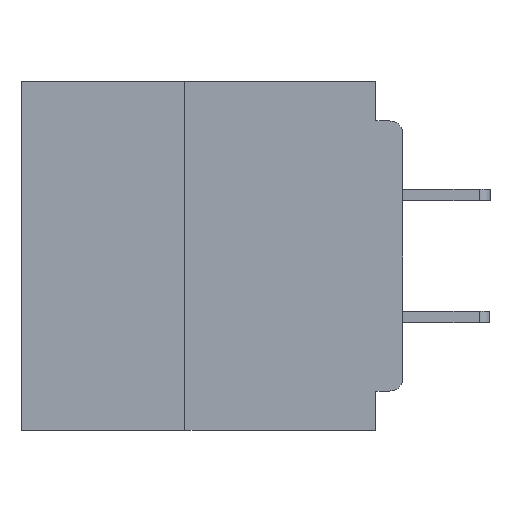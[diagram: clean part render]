
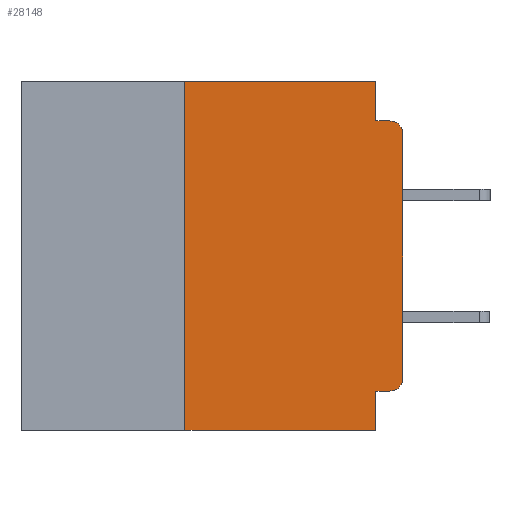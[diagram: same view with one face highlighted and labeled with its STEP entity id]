
A CAD part, left-side view. The second image highlights one B-rep face of the part: STEP entity #28148.
In plain terms, the highlighted planar face has unit normal (-1, 0, 0).
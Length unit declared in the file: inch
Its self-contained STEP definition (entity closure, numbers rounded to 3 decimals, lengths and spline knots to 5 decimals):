
#77 = VECTOR ( 'NONE', #42183, 39.37008 ) ;
#460 = LINE ( 'NONE', #24441, #40232 ) ;
#574 = CARTESIAN_POINT ( 'NONE',  ( 0., 0.031, -0.045 ) ) ;
#2517 = ORIENTED_EDGE ( 'NONE', *, *, #39709, .F. ) ;
#3654 = EDGE_LOOP ( 'NONE', ( #5285, #47737, #23604, #25950, #2517, #32413, #17317, #17014, #15145, #31941 ) ) ;
#4628 = VECTOR ( 'NONE', #46398, 39.37008 ) ;
#5285 = ORIENTED_EDGE ( 'NONE', *, *, #34865, .T. ) ;
#6125 = EDGE_CURVE ( 'NONE', #38846, #48118, #34156, .T. ) ;
#6156 = AXIS2_PLACEMENT_3D ( 'NONE', #8438, #35340, #12308 ) ;
#7947 = FACE_OUTER_BOUND ( 'NONE', #3654, .T. ) ;
#7994 = AXIS2_PLACEMENT_3D ( 'NONE', #38970, #15963, #42852 ) ;
#8438 = CARTESIAN_POINT ( 'NONE',  ( 0., 0.015, -0.06 ) ) ;
#9023 = LINE ( 'NONE', #13300, #45116 ) ;
#9073 = EDGE_CURVE ( 'NONE', #45238, #28846, #9153, .T. ) ;
#9153 = LINE ( 'NONE', #19174, #28459 ) ;
#9970 = LINE ( 'NONE', #39546, #30449 ) ;
#12308 = DIRECTION ( 'NONE',  ( 0., 0., -1. ) ) ;
#13300 = CARTESIAN_POINT ( 'NONE',  ( 0., 0.031, 0. ) ) ;
#13889 = EDGE_CURVE ( 'NONE', #40724, #48118, #30851, .T. ) ;
#14187 = CIRCLE ( 'NONE', #7994, 0.015 ) ;
#14848 = CARTESIAN_POINT ( 'NONE',  ( 0., 0.25, 0. ) ) ;
#15145 = ORIENTED_EDGE ( 'NONE', *, *, #35823, .F. ) ;
#15295 = CARTESIAN_POINT ( 'NONE',  ( 0., 0.437, -0.4 ) ) ;
#15963 = DIRECTION ( 'NONE',  ( -1., 0., 0. ) ) ;
#16493 = LINE ( 'NONE', #18394, #34532 ) ;
#16531 = DIRECTION ( 'NONE',  ( 0., 0., 1. ) ) ;
#16732 = VERTEX_POINT ( 'NONE', #42373 ) ;
#17014 = ORIENTED_EDGE ( 'NONE', *, *, #6125, .F. ) ;
#17317 = ORIENTED_EDGE ( 'NONE', *, *, #13889, .T. ) ;
#17797 = EDGE_CURVE ( 'NONE', #33479, #45098, #14187, .T. ) ;
#18394 = CARTESIAN_POINT ( 'NONE',  ( 0., 0., -0.355 ) ) ;
#19174 = CARTESIAN_POINT ( 'NONE',  ( 0., 0., -0.045 ) ) ;
#19525 = CARTESIAN_POINT ( 'NONE',  ( 0., 0.031, -0.4 ) ) ;
#19835 = CARTESIAN_POINT ( 'NONE',  ( 0., 0.437, 0. ) ) ;
#21661 = EDGE_CURVE ( 'NONE', #40724, #37680, #460, .T. ) ;
#23061 = DIRECTION ( 'NONE',  ( 0., -1., 0. ) ) ;
#23138 = LINE ( 'NONE', #32837, #30924 ) ;
#23604 = ORIENTED_EDGE ( 'NONE', *, *, #9073, .F. ) ;
#23722 = PLANE ( 'NONE',  #29336 ) ;
#23829 = CARTESIAN_POINT ( 'NONE',  ( 0., 0.015, -0.045 ) ) ;
#24223 = EDGE_CURVE ( 'NONE', #44104, #45238, #9023, .T. ) ;
#24441 = CARTESIAN_POINT ( 'NONE',  ( 0., 0.25, -0.4 ) ) ;
#25950 = ORIENTED_EDGE ( 'NONE', *, *, #24223, .F. ) ;
#27590 = DIRECTION ( 'NONE',  ( 0., 0., -1. ) ) ;
#28148 = ADVANCED_FACE ( 'NONE', ( #7947 ), #23722, .F. ) ;
#28459 = VECTOR ( 'NONE', #23061, 39.37008 ) ;
#28846 = VERTEX_POINT ( 'NONE', #23829 ) ;
#29336 = AXIS2_PLACEMENT_3D ( 'NONE', #19835, #38962, #27590 ) ;
#30449 = VECTOR ( 'NONE', #16531, 39.37008 ) ;
#30680 = EDGE_CURVE ( 'NONE', #16732, #28846, #40246, .T. ) ;
#30851 = LINE ( 'NONE', #15295, #77 ) ;
#30924 = VECTOR ( 'NONE', #36687, 39.37008 ) ;
#31941 = ORIENTED_EDGE ( 'NONE', *, *, #17797, .T. ) ;
#32157 = DIRECTION ( 'NONE',  ( 0., 0., 1. ) ) ;
#32413 = ORIENTED_EDGE ( 'NONE', *, *, #21661, .F. ) ;
#32837 = CARTESIAN_POINT ( 'NONE',  ( 0., 0.437, 0. ) ) ;
#33479 = VERTEX_POINT ( 'NONE', #43032 ) ;
#34156 = LINE ( 'NONE', #19525, #4628 ) ;
#34532 = VECTOR ( 'NONE', #41398, 39.37008 ) ;
#34865 = EDGE_CURVE ( 'NONE', #45098, #16732, #9970, .T. ) ;
#35074 = CARTESIAN_POINT ( 'NONE',  ( 0., 0.25, -0.4 ) ) ;
#35340 = DIRECTION ( 'NONE',  ( -1., 0., 0. ) ) ;
#35823 = EDGE_CURVE ( 'NONE', #33479, #38846, #16493, .T. ) ;
#36687 = DIRECTION ( 'NONE',  ( 0., -1., 0. ) ) ;
#37680 = VERTEX_POINT ( 'NONE', #14848 ) ;
#38235 = CARTESIAN_POINT ( 'NONE',  ( 0., 0.031, -0.355 ) ) ;
#38846 = VERTEX_POINT ( 'NONE', #38235 ) ;
#38962 = DIRECTION ( 'NONE',  ( 1., 0., 0. ) ) ;
#38970 = CARTESIAN_POINT ( 'NONE',  ( 0., 0.015, -0.34 ) ) ;
#39546 = CARTESIAN_POINT ( 'NONE',  ( 0., 0., 0. ) ) ;
#39709 = EDGE_CURVE ( 'NONE', #37680, #44104, #23138, .T. ) ;
#40005 = DIRECTION ( 'NONE',  ( 0., 0., -1. ) ) ;
#40232 = VECTOR ( 'NONE', #32157, 39.37008 ) ;
#40246 = CIRCLE ( 'NONE', #6156, 0.015 ) ;
#40724 = VERTEX_POINT ( 'NONE', #35074 ) ;
#41398 = DIRECTION ( 'NONE',  ( 0., 1., 0. ) ) ;
#41564 = CARTESIAN_POINT ( 'NONE',  ( 0., 0.031, -0.4 ) ) ;
#42183 = DIRECTION ( 'NONE',  ( 0., -1., 0. ) ) ;
#42373 = CARTESIAN_POINT ( 'NONE',  ( 0., 0., -0.06 ) ) ;
#42852 = DIRECTION ( 'NONE',  ( 0., 0., -1. ) ) ;
#42934 = CARTESIAN_POINT ( 'NONE',  ( 0., 0.031, 0. ) ) ;
#43032 = CARTESIAN_POINT ( 'NONE',  ( 0., 0.015, -0.355 ) ) ;
#44104 = VERTEX_POINT ( 'NONE', #42934 ) ;
#45098 = VERTEX_POINT ( 'NONE', #45874 ) ;
#45116 = VECTOR ( 'NONE', #40005, 39.37008 ) ;
#45238 = VERTEX_POINT ( 'NONE', #574 ) ;
#45874 = CARTESIAN_POINT ( 'NONE',  ( 0., 0., -0.34 ) ) ;
#46398 = DIRECTION ( 'NONE',  ( 0., 0., -1. ) ) ;
#47737 = ORIENTED_EDGE ( 'NONE', *, *, #30680, .T. ) ;
#48118 = VERTEX_POINT ( 'NONE', #41564 ) ;
